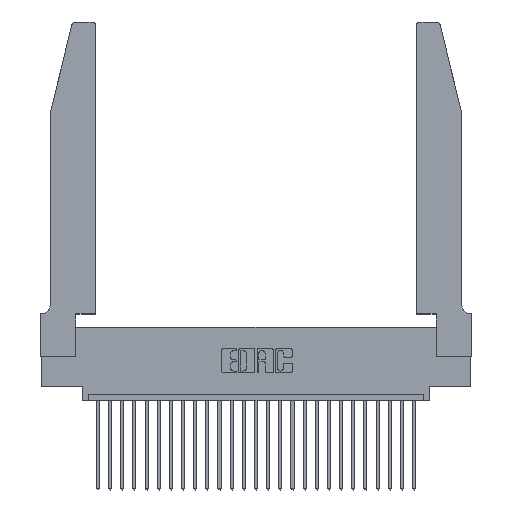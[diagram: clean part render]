
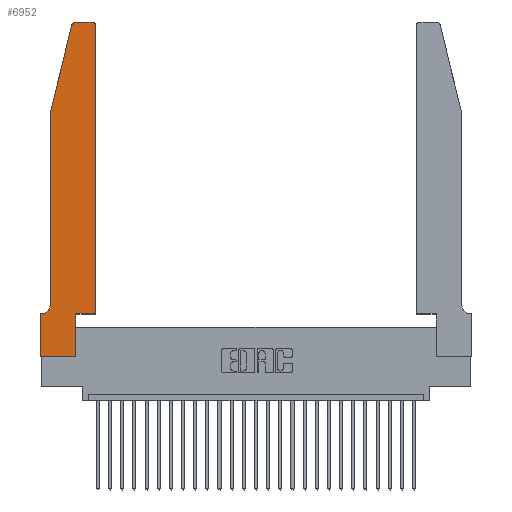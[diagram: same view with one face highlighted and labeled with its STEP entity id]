
A CAD part, top view. The second image highlights one B-rep face of the part: STEP entity #6952.
In plain terms, the highlighted planar face has unit normal (0, 0, 1).
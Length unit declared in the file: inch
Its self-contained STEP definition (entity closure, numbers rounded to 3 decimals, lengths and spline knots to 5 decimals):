
#103 = AXIS2_PLACEMENT_3D ( 'NONE', #16233, #7882, #27023 ) ;
#1150 = DIRECTION ( 'NONE',  ( 0., 1., 0. ) ) ;
#1207 = VERTEX_POINT ( 'NONE', #10253 ) ;
#2457 = EDGE_CURVE ( 'NONE', #13807, #21274, #15256, .T. ) ;
#2584 = VECTOR ( 'NONE', #21472, 39.37008 ) ;
#3230 = ORIENTED_EDGE ( 'NONE', *, *, #19981, .T. ) ;
#3292 = CARTESIAN_POINT ( 'NONE',  ( 0.4505, 0.35, 0.37 ) ) ;
#3325 = AXIS2_PLACEMENT_3D ( 'NONE', #4275, #10466, #27273 ) ;
#4018 = DIRECTION ( 'NONE',  ( 0., 0., -1. ) ) ;
#4149 = VECTOR ( 'NONE', #4935, 39.37008 ) ;
#4210 = LINE ( 'NONE', #6826, #2584 ) ;
#4275 = CARTESIAN_POINT ( 'NONE',  ( 0.284, 2.72, 0.37 ) ) ;
#4306 = EDGE_CURVE ( 'NONE', #5455, #16813, #22716, .T. ) ;
#4463 = LINE ( 'NONE', #11204, #4149 ) ;
#4665 = CIRCLE ( 'NONE', #103, 0.03 ) ;
#4746 = DIRECTION ( 'NONE',  ( 1., 0., 0. ) ) ;
#4935 = DIRECTION ( 'NONE',  ( 0., -1., 0. ) ) ;
#5195 = EDGE_CURVE ( 'NONE', #16813, #26106, #9510, .T. ) ;
#5203 = VERTEX_POINT ( 'NONE', #3292 ) ;
#5209 = CARTESIAN_POINT ( 'NONE',  ( 0.0755, 2., 0.37 ) ) ;
#5394 = CARTESIAN_POINT ( 'NONE',  ( 0., 0., 0.37 ) ) ;
#5455 = VERTEX_POINT ( 'NONE', #14665 ) ;
#5820 = CARTESIAN_POINT ( 'NONE',  ( 0., 0., 0.37 ) ) ;
#5878 = EDGE_CURVE ( 'NONE', #15305, #19259, #4210, .T. ) ;
#6189 = ORIENTED_EDGE ( 'NONE', *, *, #25938, .T. ) ;
#6246 = CARTESIAN_POINT ( 'NONE',  ( 0.4505, 0.35, 0.37 ) ) ;
#6763 = PLANE ( 'NONE',  #20886 ) ;
#6826 = CARTESIAN_POINT ( 'NONE',  ( 0.2605, 2.75, 0.37 ) ) ;
#6920 = DIRECTION ( 'NONE',  ( 1., 0., 0. ) ) ;
#6952 = ADVANCED_FACE ( 'NONE', ( #26215 ), #6763, .T. ) ;
#6957 = LINE ( 'NONE', #11573, #21119 ) ;
#7222 = VECTOR ( 'NONE', #9924, 39.37008 ) ;
#7810 = ORIENTED_EDGE ( 'NONE', *, *, #5195, .T. ) ;
#7882 = DIRECTION ( 'NONE',  ( 0., 0., 1. ) ) ;
#8610 = CARTESIAN_POINT ( 'NONE',  ( 0.0755, 2., 0.37 ) ) ;
#8732 = EDGE_CURVE ( 'NONE', #5203, #20185, #12407, .T. ) ;
#9218 = CARTESIAN_POINT ( 'NONE',  ( 0., 0., 0.37 ) ) ;
#9266 = DIRECTION ( 'NONE',  ( 1., 0., 0. ) ) ;
#9432 = ORIENTED_EDGE ( 'NONE', *, *, #18259, .T. ) ;
#9510 = LINE ( 'NONE', #5394, #7222 ) ;
#9540 = DIRECTION ( 'NONE',  ( -0.239, -0.971, 0. ) ) ;
#9755 = CARTESIAN_POINT ( 'NONE',  ( 0.4505, 2.72, 0.37 ) ) ;
#9886 = EDGE_CURVE ( 'NONE', #19259, #13807, #21930, .T. ) ;
#9924 = DIRECTION ( 'NONE',  ( 0., -1., 0. ) ) ;
#10078 = ORIENTED_EDGE ( 'NONE', *, *, #15294, .T. ) ;
#10253 = CARTESIAN_POINT ( 'NONE',  ( 0.2865, 0.35, 0.37 ) ) ;
#10466 = DIRECTION ( 'NONE',  ( 0., 0., 1. ) ) ;
#11204 = CARTESIAN_POINT ( 'NONE',  ( 0.0755, 2., 0.37 ) ) ;
#11573 = CARTESIAN_POINT ( 'NONE',  ( 0.4505, 0.35, 0.37 ) ) ;
#11633 = ORIENTED_EDGE ( 'NONE', *, *, #9886, .T. ) ;
#12082 = VECTOR ( 'NONE', #21616, 39.37008 ) ;
#12407 = LINE ( 'NONE', #6246, #12082 ) ;
#12501 = CARTESIAN_POINT ( 'NONE',  ( 0.0055, 0.42, 0.37 ) ) ;
#12936 = ORIENTED_EDGE ( 'NONE', *, *, #5878, .T. ) ;
#13401 = ORIENTED_EDGE ( 'NONE', *, *, #15380, .T. ) ;
#13754 = CARTESIAN_POINT ( 'NONE',  ( 0.2865, 0.35, 0.37 ) ) ;
#13807 = VERTEX_POINT ( 'NONE', #20781 ) ;
#14611 = ORIENTED_EDGE ( 'NONE', *, *, #8732, .T. ) ;
#14665 = CARTESIAN_POINT ( 'NONE',  ( 0.0055, 0.35, 0.37 ) ) ;
#15042 = EDGE_LOOP ( 'NONE', ( #12936, #11633, #23616, #22975, #3230, #22777, #7810, #9432, #6189, #10078, #14611, #13401 ) ) ;
#15256 = LINE ( 'NONE', #5209, #15896 ) ;
#15294 = EDGE_CURVE ( 'NONE', #1207, #5203, #6957, .T. ) ;
#15305 = VERTEX_POINT ( 'NONE', #24040 ) ;
#15380 = EDGE_CURVE ( 'NONE', #20185, #15305, #4665, .T. ) ;
#15428 = CARTESIAN_POINT ( 'NONE',  ( 0., 0.35, 0.37 ) ) ;
#15429 = VECTOR ( 'NONE', #6920, 39.37008 ) ;
#15890 = CARTESIAN_POINT ( 'NONE',  ( 0.0755, 0.42, 0.37 ) ) ;
#15896 = VECTOR ( 'NONE', #9540, 39.37008 ) ;
#15981 = CARTESIAN_POINT ( 'NONE',  ( 0.2865, 0., 0.37 ) ) ;
#16233 = CARTESIAN_POINT ( 'NONE',  ( 0.4205, 2.72, 0.37 ) ) ;
#16813 = VERTEX_POINT ( 'NONE', #18557 ) ;
#17787 = VECTOR ( 'NONE', #22391, 39.37008 ) ;
#18176 = CARTESIAN_POINT ( 'NONE',  ( 0.0755, 0.35, 0.37 ) ) ;
#18259 = EDGE_CURVE ( 'NONE', #26106, #27180, #21999, .T. ) ;
#18557 = CARTESIAN_POINT ( 'NONE',  ( 0., 0.35, 0.37 ) ) ;
#19259 = VERTEX_POINT ( 'NONE', #21262 ) ;
#19370 = LINE ( 'NONE', #13754, #26927 ) ;
#19981 = EDGE_CURVE ( 'NONE', #20314, #5455, #23152, .T. ) ;
#20185 = VERTEX_POINT ( 'NONE', #9755 ) ;
#20314 = VERTEX_POINT ( 'NONE', #15890 ) ;
#20567 = EDGE_CURVE ( 'NONE', #21274, #20314, #4463, .T. ) ;
#20781 = CARTESIAN_POINT ( 'NONE',  ( 0.25487, 2.72718, 0.37 ) ) ;
#20886 = AXIS2_PLACEMENT_3D ( 'NONE', #15428, #23843, #4746 ) ;
#21119 = VECTOR ( 'NONE', #9266, 39.37008 ) ;
#21262 = CARTESIAN_POINT ( 'NONE',  ( 0.284, 2.75, 0.37 ) ) ;
#21274 = VERTEX_POINT ( 'NONE', #8610 ) ;
#21472 = DIRECTION ( 'NONE',  ( -1., 0., 0. ) ) ;
#21616 = DIRECTION ( 'NONE',  ( 0., 1., 0. ) ) ;
#21930 = CIRCLE ( 'NONE', #3325, 0.03 ) ;
#21999 = LINE ( 'NONE', #9218, #15429 ) ;
#22264 = AXIS2_PLACEMENT_3D ( 'NONE', #12501, #4018, #22819 ) ;
#22391 = DIRECTION ( 'NONE',  ( -1., 0., 0. ) ) ;
#22716 = LINE ( 'NONE', #18176, #17787 ) ;
#22777 = ORIENTED_EDGE ( 'NONE', *, *, #4306, .T. ) ;
#22819 = DIRECTION ( 'NONE',  ( -1., 0., 0. ) ) ;
#22975 = ORIENTED_EDGE ( 'NONE', *, *, #20567, .T. ) ;
#23152 = CIRCLE ( 'NONE', #22264, 0.07 ) ;
#23616 = ORIENTED_EDGE ( 'NONE', *, *, #2457, .T. ) ;
#23843 = DIRECTION ( 'NONE',  ( 0., 0., 1. ) ) ;
#24040 = CARTESIAN_POINT ( 'NONE',  ( 0.4205, 2.75, 0.37 ) ) ;
#25938 = EDGE_CURVE ( 'NONE', #27180, #1207, #19370, .T. ) ;
#26106 = VERTEX_POINT ( 'NONE', #5820 ) ;
#26215 = FACE_OUTER_BOUND ( 'NONE', #15042, .T. ) ;
#26927 = VECTOR ( 'NONE', #1150, 39.37008 ) ;
#27023 = DIRECTION ( 'NONE',  ( 1., 0., 0. ) ) ;
#27180 = VERTEX_POINT ( 'NONE', #15981 ) ;
#27273 = DIRECTION ( 'NONE',  ( 1., 0., 0. ) ) ;
